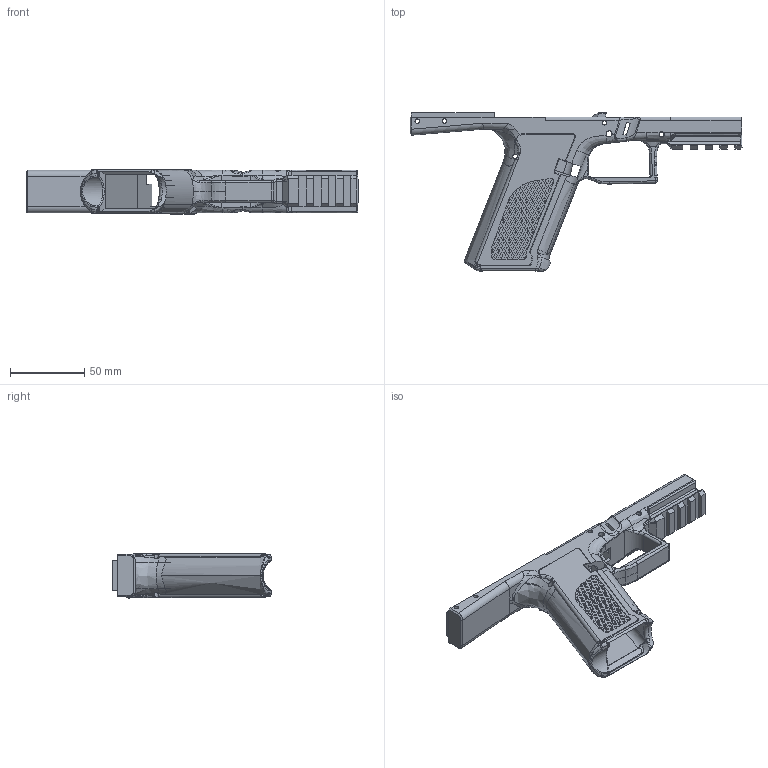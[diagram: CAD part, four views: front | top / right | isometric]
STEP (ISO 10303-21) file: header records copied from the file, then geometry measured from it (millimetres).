
FILE_DESCRIPTION(/* description */ (''),/* implementation_level */ '2;1');
FILE_NAME(/* name */ 'USW Frame.step',/* time_stamp */ '2023-02-14T18:49:50-07:00',/* author */ (''),/* organization */ (''),/* preprocessor_version */ 'ST-DEVELOPER v19.2',/* originating_system */ 'Autodesk Translation Framework v11.17.0.187',/* authorisation */ '');
FILE_SCHEMA (('AUTOMOTIVE_DESIGN { 1 0 10303 214 3 1 1 }'));
Products named in the file (1): G19X
Bounding box: 223.42 x 106.5 x 30.25 mm (x, y, z)
Volume: 110630.4 mm3; surface area: 53871.6 mm2
Topology: 1 solids, 1 shells, 2371 faces, 6149 edges, 3967 vertices
Faces by surface type: bspline 1181, plane 909, cylinder 219, torus 43, sphere 12, cone 7
Full cylindrical faces by diameter (mm): 2 x1, 3 x4, 3.2 x2, 4 x2
Entity records: 101180 total; most frequent: CARTESIAN_POINT 52709, ORIENTED_EDGE 12264, DIRECTION 6849, EDGE_CURVE 6132, VERTEX_POINT 3968, LINE 2999, VECTOR 2999, EDGE_LOOP 2610
